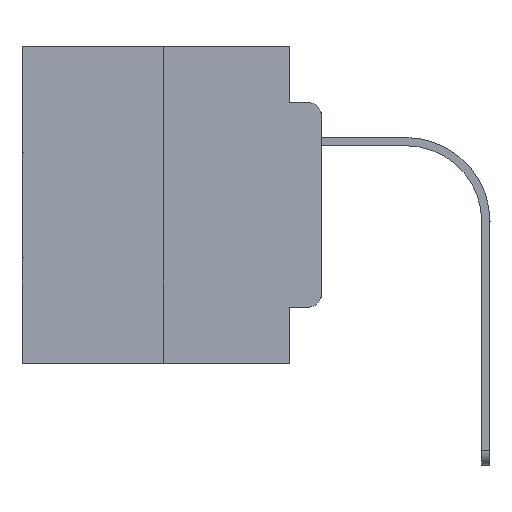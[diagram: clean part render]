
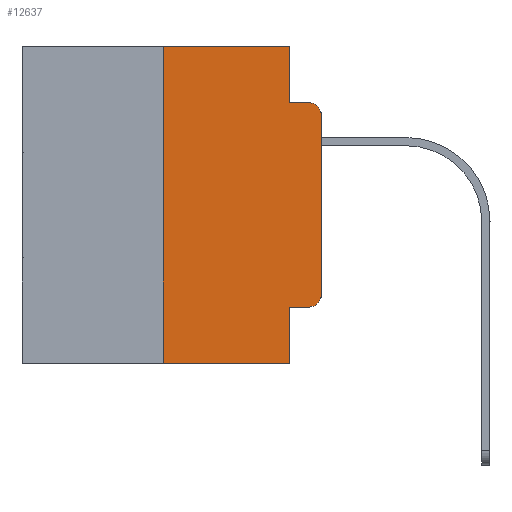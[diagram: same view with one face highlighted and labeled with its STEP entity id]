
A CAD part, left-side view. The second image highlights one B-rep face of the part: STEP entity #12637.
In plain terms, the highlighted planar face has unit normal (-1, 0, 0).
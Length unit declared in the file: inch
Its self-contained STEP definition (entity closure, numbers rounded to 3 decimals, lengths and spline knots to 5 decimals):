
#174 = LINE ( 'NONE', #13799, #6368 ) ;
#280 = CARTESIAN_POINT ( 'NONE',  ( 0., 0.051, -0.0885 ) ) ;
#305 = CARTESIAN_POINT ( 'NONE',  ( 0., 0.02, -0.0885 ) ) ;
#852 = VERTEX_POINT ( 'NONE', #23763 ) ;
#1091 = DIRECTION ( 'NONE',  ( -1., 0., 0. ) ) ;
#1137 = VERTEX_POINT ( 'NONE', #12119 ) ;
#1391 = VERTEX_POINT ( 'NONE', #21593 ) ;
#1519 = VECTOR ( 'NONE', #5688, 39.37008 ) ;
#1521 = DIRECTION ( 'NONE',  ( 0., 0., -1. ) ) ;
#1703 = LINE ( 'NONE', #14481, #1519 ) ;
#1726 = EDGE_LOOP ( 'NONE', ( #18091, #12463, #25758, #16605, #5708, #9346, #14229, #17787, #16702, #9691 ) ) ;
#2036 = CARTESIAN_POINT ( 'NONE',  ( 0., 0., -0.3915 ) ) ;
#2287 = CARTESIAN_POINT ( 'NONE',  ( 0., 0.02, -0.3915 ) ) ;
#2347 = AXIS2_PLACEMENT_3D ( 'NONE', #20516, #1091, #27341 ) ;
#2727 = VECTOR ( 'NONE', #1521, 39.37008 ) ;
#3486 = DIRECTION ( 'NONE',  ( 1., 0., 0. ) ) ;
#3924 = LINE ( 'NONE', #16832, #2727 ) ;
#4230 = EDGE_CURVE ( 'NONE', #14946, #7394, #3924, .T. ) ;
#4597 = VERTEX_POINT ( 'NONE', #23289 ) ;
#4894 = CARTESIAN_POINT ( 'NONE',  ( 0., 0.473, 0. ) ) ;
#5036 = DIRECTION ( 'NONE',  ( 0., 0., -1. ) ) ;
#5115 = DIRECTION ( 'NONE',  ( 0., -1., 0. ) ) ;
#5207 = CIRCLE ( 'NONE', #25611, 0.02 ) ;
#5513 = EDGE_CURVE ( 'NONE', #26863, #4597, #21358, .T. ) ;
#5688 = DIRECTION ( 'NONE',  ( 0., 0., 1. ) ) ;
#5708 = ORIENTED_EDGE ( 'NONE', *, *, #14152, .F. ) ;
#6246 = DIRECTION ( 'NONE',  ( 0., 0., -1. ) ) ;
#6368 = VECTOR ( 'NONE', #8842, 39.37008 ) ;
#7394 = VERTEX_POINT ( 'NONE', #280 ) ;
#8333 = CARTESIAN_POINT ( 'NONE',  ( 0., 0.051, -0.4115 ) ) ;
#8634 = VECTOR ( 'NONE', #9643, 39.37008 ) ;
#8842 = DIRECTION ( 'NONE',  ( 0., 0., 1. ) ) ;
#9109 = LINE ( 'NONE', #24833, #9668 ) ;
#9346 = ORIENTED_EDGE ( 'NONE', *, *, #24799, .F. ) ;
#9643 = DIRECTION ( 'NONE',  ( 0., 0., -1. ) ) ;
#9668 = VECTOR ( 'NONE', #5115, 39.37008 ) ;
#9691 = ORIENTED_EDGE ( 'NONE', *, *, #17106, .T. ) ;
#10023 = VERTEX_POINT ( 'NONE', #2036 ) ;
#10487 = VECTOR ( 'NONE', #10592, 39.37008 ) ;
#10592 = DIRECTION ( 'NONE',  ( 0., -1., 0. ) ) ;
#10745 = LINE ( 'NONE', #25504, #16038 ) ;
#10944 = DIRECTION ( 'NONE',  ( -1., 0., 0. ) ) ;
#12119 = CARTESIAN_POINT ( 'NONE',  ( 0., 0.25, -0.5 ) ) ;
#12162 = VERTEX_POINT ( 'NONE', #305 ) ;
#12463 = ORIENTED_EDGE ( 'NONE', *, *, #26787, .T. ) ;
#12637 = ADVANCED_FACE ( 'NONE', ( #19942 ), #24343, .F. ) ;
#13519 = EDGE_CURVE ( 'NONE', #1137, #852, #9109, .T. ) ;
#13643 = EDGE_CURVE ( 'NONE', #10023, #1391, #1703, .T. ) ;
#13762 = LINE ( 'NONE', #22408, #8634 ) ;
#13799 = CARTESIAN_POINT ( 'NONE',  ( 0., 0.25, 0. ) ) ;
#14152 = EDGE_CURVE ( 'NONE', #20664, #14946, #10745, .T. ) ;
#14156 = CARTESIAN_POINT ( 'NONE',  ( 0., 0.051, 0. ) ) ;
#14229 = ORIENTED_EDGE ( 'NONE', *, *, #13519, .T. ) ;
#14481 = CARTESIAN_POINT ( 'NONE',  ( 0., 0., 0. ) ) ;
#14946 = VERTEX_POINT ( 'NONE', #14156 ) ;
#15398 = DIRECTION ( 'NONE',  ( 0., -1., 0. ) ) ;
#15473 = CIRCLE ( 'NONE', #2347, 0.02 ) ;
#15813 = CARTESIAN_POINT ( 'NONE',  ( 0., 0.051, -0.0885 ) ) ;
#16038 = VECTOR ( 'NONE', #21798, 39.37008 ) ;
#16605 = ORIENTED_EDGE ( 'NONE', *, *, #4230, .F. ) ;
#16702 = ORIENTED_EDGE ( 'NONE', *, *, #5513, .T. ) ;
#16832 = CARTESIAN_POINT ( 'NONE',  ( 0., 0.051, 0. ) ) ;
#16971 = CARTESIAN_POINT ( 'NONE',  ( 0., 0.051, -0.4115 ) ) ;
#17106 = EDGE_CURVE ( 'NONE', #4597, #10023, #5207, .T. ) ;
#17787 = ORIENTED_EDGE ( 'NONE', *, *, #25372, .F. ) ;
#18091 = ORIENTED_EDGE ( 'NONE', *, *, #13643, .T. ) ;
#18819 = VECTOR ( 'NONE', #15398, 39.37008 ) ;
#19366 = EDGE_CURVE ( 'NONE', #7394, #12162, #26603, .T. ) ;
#19942 = FACE_OUTER_BOUND ( 'NONE', #1726, .T. ) ;
#20516 = CARTESIAN_POINT ( 'NONE',  ( 0., 0.02, -0.1085 ) ) ;
#20664 = VERTEX_POINT ( 'NONE', #21535 ) ;
#21358 = LINE ( 'NONE', #8333, #10487 ) ;
#21385 = AXIS2_PLACEMENT_3D ( 'NONE', #4894, #3486, #5036 ) ;
#21535 = CARTESIAN_POINT ( 'NONE',  ( 0., 0.25, 0. ) ) ;
#21593 = CARTESIAN_POINT ( 'NONE',  ( 0., 0., -0.1085 ) ) ;
#21798 = DIRECTION ( 'NONE',  ( 0., -1., 0. ) ) ;
#22408 = CARTESIAN_POINT ( 'NONE',  ( 0., 0.051, 0. ) ) ;
#23289 = CARTESIAN_POINT ( 'NONE',  ( 0., 0.02, -0.4115 ) ) ;
#23763 = CARTESIAN_POINT ( 'NONE',  ( 0., 0.051, -0.5 ) ) ;
#24343 = PLANE ( 'NONE',  #21385 ) ;
#24799 = EDGE_CURVE ( 'NONE', #1137, #20664, #174, .T. ) ;
#24833 = CARTESIAN_POINT ( 'NONE',  ( 0., 0.473, -0.5 ) ) ;
#25372 = EDGE_CURVE ( 'NONE', #26863, #852, #13762, .T. ) ;
#25504 = CARTESIAN_POINT ( 'NONE',  ( 0., 0.473, 0. ) ) ;
#25611 = AXIS2_PLACEMENT_3D ( 'NONE', #2287, #10944, #6246 ) ;
#25758 = ORIENTED_EDGE ( 'NONE', *, *, #19366, .F. ) ;
#26603 = LINE ( 'NONE', #15813, #18819 ) ;
#26787 = EDGE_CURVE ( 'NONE', #1391, #12162, #15473, .T. ) ;
#26863 = VERTEX_POINT ( 'NONE', #16971 ) ;
#27341 = DIRECTION ( 'NONE',  ( 0., 0., -1. ) ) ;
